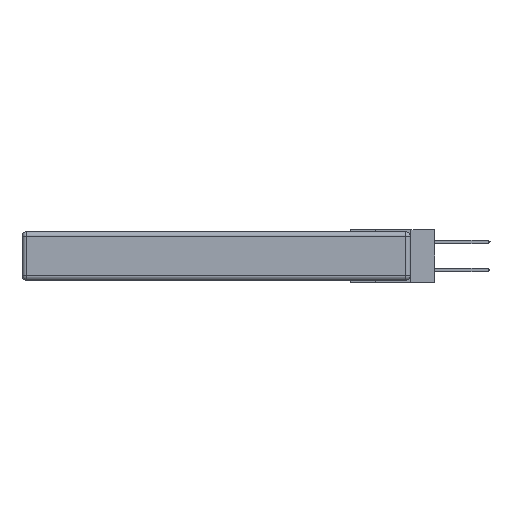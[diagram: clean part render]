
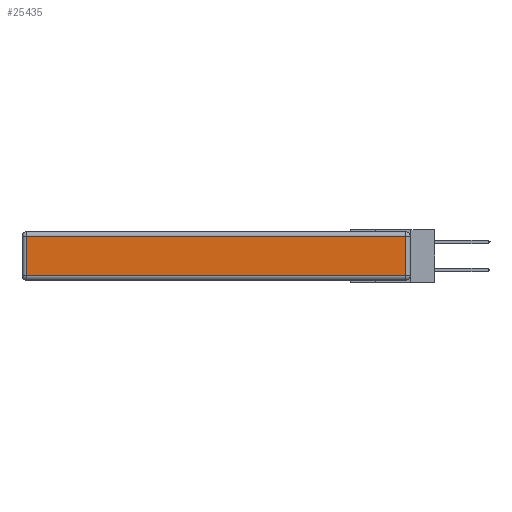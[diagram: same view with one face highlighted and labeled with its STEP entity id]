
A CAD part, left-side view. The second image highlights one B-rep face of the part: STEP entity #25435.
In plain terms, the highlighted planar face has unit normal (-1, 0, 0).
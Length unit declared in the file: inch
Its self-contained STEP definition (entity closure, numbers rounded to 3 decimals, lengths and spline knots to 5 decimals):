
#1776 = ORIENTED_EDGE ( 'NONE', *, *, #25298, .T. ) ;
#1926 = CARTESIAN_POINT ( 'NONE',  ( 0., 2.72, -0.313 ) ) ;
#2049 = PLANE ( 'NONE',  #25841 ) ;
#2682 = DIRECTION ( 'NONE',  ( 0., -1., 0. ) ) ;
#4154 = VERTEX_POINT ( 'NONE', #28897 ) ;
#4295 = ORIENTED_EDGE ( 'NONE', *, *, #5179, .T. ) ;
#4377 = VECTOR ( 'NONE', #26397, 39.37008 ) ;
#5179 = EDGE_CURVE ( 'NONE', #4154, #30379, #7522, .T. ) ;
#6978 = LINE ( 'NONE', #16500, #8555 ) ;
#7522 = LINE ( 'NONE', #31635, #4377 ) ;
#8555 = VECTOR ( 'NONE', #9022, 39.37008 ) ;
#8880 = FACE_OUTER_BOUND ( 'NONE', #13115, .T. ) ;
#9022 = DIRECTION ( 'NONE',  ( 0., 0., 1. ) ) ;
#9343 = DIRECTION ( 'NONE',  ( -1., 0., 0. ) ) ;
#10081 = LINE ( 'NONE', #14968, #15884 ) ;
#11321 = ORIENTED_EDGE ( 'NONE', *, *, #30381, .T. ) ;
#12518 = CARTESIAN_POINT ( 'NONE',  ( 0., 0.03, -0.313 ) ) ;
#13115 = EDGE_LOOP ( 'NONE', ( #1776, #20530, #11321, #4295 ) ) ;
#13865 = VERTEX_POINT ( 'NONE', #12518 ) ;
#14968 = CARTESIAN_POINT ( 'NONE',  ( 0., 0., -0.313 ) ) ;
#15737 = EDGE_CURVE ( 'NONE', #13865, #23877, #6978, .T. ) ;
#15884 = VECTOR ( 'NONE', #2682, 39.37008 ) ;
#16444 = CARTESIAN_POINT ( 'NONE',  ( 0., 0.03, -0.03 ) ) ;
#16500 = CARTESIAN_POINT ( 'NONE',  ( 0., 0.03, -0.343 ) ) ;
#17704 = DIRECTION ( 'NONE',  ( 0., 0., 1. ) ) ;
#19328 = CARTESIAN_POINT ( 'NONE',  ( 0., 0., -0.343 ) ) ;
#20530 = ORIENTED_EDGE ( 'NONE', *, *, #15737, .T. ) ;
#20775 = LINE ( 'NONE', #29473, #28588 ) ;
#23877 = VERTEX_POINT ( 'NONE', #16444 ) ;
#25298 = EDGE_CURVE ( 'NONE', #30379, #13865, #10081, .T. ) ;
#25435 = ADVANCED_FACE ( 'NONE', ( #8880 ), #2049, .T. ) ;
#25841 = AXIS2_PLACEMENT_3D ( 'NONE', #19328, #9343, #17704 ) ;
#26397 = DIRECTION ( 'NONE',  ( 0., 0., -1. ) ) ;
#26983 = DIRECTION ( 'NONE',  ( 0., 1., 0. ) ) ;
#28588 = VECTOR ( 'NONE', #26983, 39.37008 ) ;
#28897 = CARTESIAN_POINT ( 'NONE',  ( 0., 2.72, -0.03 ) ) ;
#29473 = CARTESIAN_POINT ( 'NONE',  ( 0., 2.75, -0.03 ) ) ;
#30379 = VERTEX_POINT ( 'NONE', #1926 ) ;
#30381 = EDGE_CURVE ( 'NONE', #23877, #4154, #20775, .T. ) ;
#31635 = CARTESIAN_POINT ( 'NONE',  ( 0., 2.72, -0.343 ) ) ;
